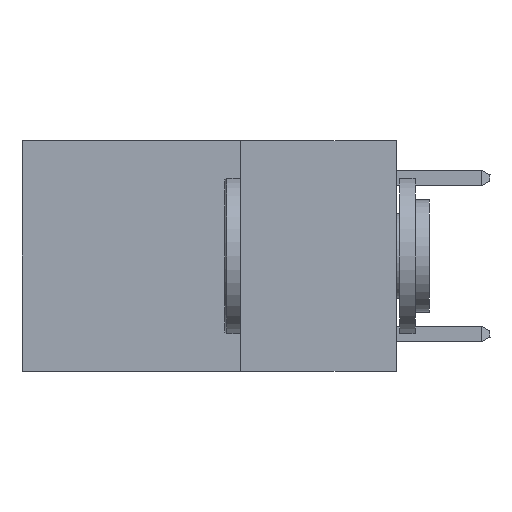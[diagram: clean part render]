
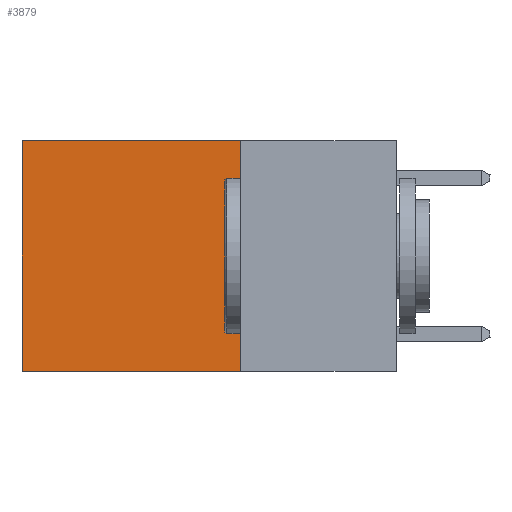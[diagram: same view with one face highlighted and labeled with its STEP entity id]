
A CAD part, left-side view. The second image highlights one B-rep face of the part: STEP entity #3879.
In plain terms, the highlighted planar face has unit normal (-1, 0, 0).
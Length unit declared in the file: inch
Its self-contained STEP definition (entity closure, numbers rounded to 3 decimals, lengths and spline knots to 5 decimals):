
#165 = VERTEX_POINT ( 'NONE', #11278 ) ;
#845 = LINE ( 'NONE', #9840, #12434 ) ;
#887 = EDGE_CURVE ( 'NONE', #12419, #165, #5360, .T. ) ;
#1818 = CARTESIAN_POINT ( 'NONE',  ( 0.2625, 0.6, 0. ) ) ;
#1911 = DIRECTION ( 'NONE',  ( 0., 1., 0. ) ) ;
#2073 = LINE ( 'NONE', #10750, #8382 ) ;
#3799 = CARTESIAN_POINT ( 'NONE',  ( 0.2625, 0.25, 0. ) ) ;
#3873 = DIRECTION ( 'NONE',  ( 0., 1., 0. ) ) ;
#3879 = ADVANCED_FACE ( 'NONE', ( #5173 ), #13132, .F. ) ;
#4374 = ORIENTED_EDGE ( 'NONE', *, *, #13723, .T. ) ;
#4869 = EDGE_LOOP ( 'NONE', ( #5011, #7434, #10742, #4374 ) ) ;
#5011 = ORIENTED_EDGE ( 'NONE', *, *, #12858, .T. ) ;
#5173 = FACE_OUTER_BOUND ( 'NONE', #4869, .T. ) ;
#5241 = DIRECTION ( 'NONE',  ( 1., 0., 0. ) ) ;
#5303 = DIRECTION ( 'NONE',  ( 0., 0., -1. ) ) ;
#5360 = LINE ( 'NONE', #9821, #12986 ) ;
#5395 = VERTEX_POINT ( 'NONE', #12765 ) ;
#5459 = CARTESIAN_POINT ( 'NONE',  ( 0.2625, 0.25, 0. ) ) ;
#5874 = EDGE_CURVE ( 'NONE', #5395, #12419, #845, .T. ) ;
#6992 = AXIS2_PLACEMENT_3D ( 'NONE', #5459, #5241, #14446 ) ;
#7434 = ORIENTED_EDGE ( 'NONE', *, *, #887, .F. ) ;
#8382 = VECTOR ( 'NONE', #9844, 39.37008 ) ;
#8416 = LINE ( 'NONE', #3799, #10517 ) ;
#9821 = CARTESIAN_POINT ( 'NONE',  ( 0.2625, 0.25, -0.37 ) ) ;
#9840 = CARTESIAN_POINT ( 'NONE',  ( 0.2625, 0.25, 0. ) ) ;
#9844 = DIRECTION ( 'NONE',  ( 0., 0., -1. ) ) ;
#10397 = VERTEX_POINT ( 'NONE', #1818 ) ;
#10517 = VECTOR ( 'NONE', #3873, 39.37008 ) ;
#10742 = ORIENTED_EDGE ( 'NONE', *, *, #5874, .F. ) ;
#10750 = CARTESIAN_POINT ( 'NONE',  ( 0.2625, 0.6, 0. ) ) ;
#11278 = CARTESIAN_POINT ( 'NONE',  ( 0.2625, 0.6, -0.37 ) ) ;
#11952 = CARTESIAN_POINT ( 'NONE',  ( 0.2625, 0.25, -0.37 ) ) ;
#12419 = VERTEX_POINT ( 'NONE', #11952 ) ;
#12434 = VECTOR ( 'NONE', #5303, 39.37008 ) ;
#12765 = CARTESIAN_POINT ( 'NONE',  ( 0.2625, 0.25, 0. ) ) ;
#12858 = EDGE_CURVE ( 'NONE', #10397, #165, #2073, .T. ) ;
#12986 = VECTOR ( 'NONE', #1911, 39.37008 ) ;
#13132 = PLANE ( 'NONE',  #6992 ) ;
#13723 = EDGE_CURVE ( 'NONE', #5395, #10397, #8416, .T. ) ;
#14446 = DIRECTION ( 'NONE',  ( 0., 0., -1. ) ) ;
